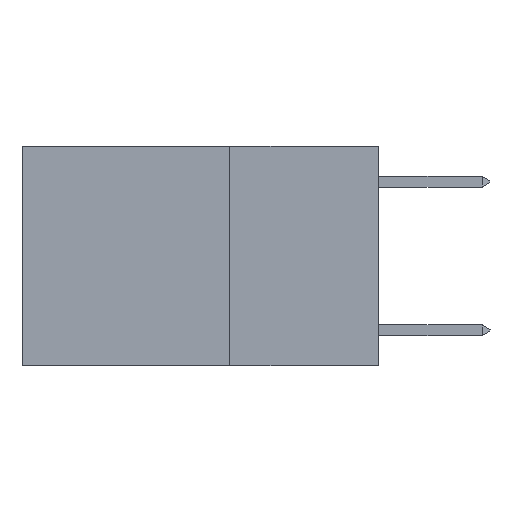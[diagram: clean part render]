
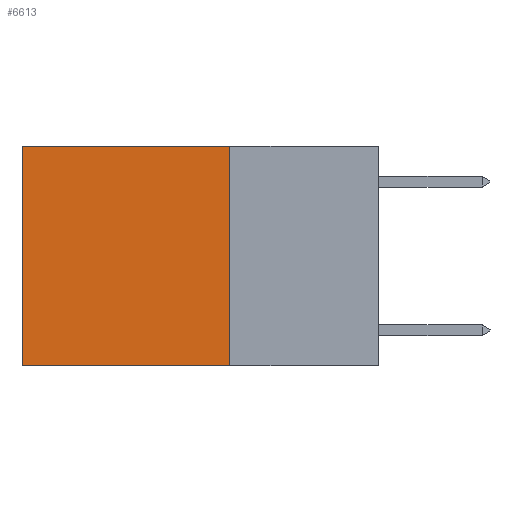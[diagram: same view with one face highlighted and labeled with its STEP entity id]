
A CAD part, left-side view. The second image highlights one B-rep face of the part: STEP entity #6613.
In plain terms, the highlighted planar face has unit normal (-1, 0, 0).
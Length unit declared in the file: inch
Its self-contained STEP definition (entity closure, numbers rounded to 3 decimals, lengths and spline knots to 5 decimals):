
#536 = EDGE_CURVE ( 'NONE', #12545, #14057, #3298, .T. ) ;
#821 = FACE_OUTER_BOUND ( 'NONE', #10818, .T. ) ;
#903 = EDGE_CURVE ( 'NONE', #1958, #10976, #19101, .T. ) ;
#1027 = EDGE_CURVE ( 'NONE', #12545, #1958, #18067, .T. ) ;
#1888 = ORIENTED_EDGE ( 'NONE', *, *, #536, .F. ) ;
#1958 = VERTEX_POINT ( 'NONE', #10747 ) ;
#2351 = ORIENTED_EDGE ( 'NONE', *, *, #14251, .F. ) ;
#2869 = VECTOR ( 'NONE', #5388, 39.37008 ) ;
#3298 = LINE ( 'NONE', #4580, #2869 ) ;
#4580 = CARTESIAN_POINT ( 'NONE',  ( 0.2625, 0.25, 0. ) ) ;
#5266 = CARTESIAN_POINT ( 'NONE',  ( 0.2625, 0.25, 0. ) ) ;
#5388 = DIRECTION ( 'NONE',  ( 0., 0., -1. ) ) ;
#6613 = ADVANCED_FACE ( 'NONE', ( #821 ), #17254, .F. ) ;
#7417 = CARTESIAN_POINT ( 'NONE',  ( 0.2625, 0.25, -0.37 ) ) ;
#7453 = ORIENTED_EDGE ( 'NONE', *, *, #1027, .T. ) ;
#10724 = AXIS2_PLACEMENT_3D ( 'NONE', #18256, #16936, #16872 ) ;
#10747 = CARTESIAN_POINT ( 'NONE',  ( 0.2625, 0.6, 0. ) ) ;
#10818 = EDGE_LOOP ( 'NONE', ( #18969, #2351, #1888, #7453 ) ) ;
#10976 = VERTEX_POINT ( 'NONE', #14517 ) ;
#11444 = CARTESIAN_POINT ( 'NONE',  ( 0.2625, 0.25, -0.37 ) ) ;
#11497 = DIRECTION ( 'NONE',  ( 0., 1., 0. ) ) ;
#11735 = CARTESIAN_POINT ( 'NONE',  ( 0.2625, 0.25, 0. ) ) ;
#11893 = DIRECTION ( 'NONE',  ( 0., 1., 0. ) ) ;
#12545 = VERTEX_POINT ( 'NONE', #5266 ) ;
#14057 = VERTEX_POINT ( 'NONE', #11444 ) ;
#14251 = EDGE_CURVE ( 'NONE', #14057, #10976, #17532, .T. ) ;
#14275 = CARTESIAN_POINT ( 'NONE',  ( 0.2625, 0.6, 0. ) ) ;
#14517 = CARTESIAN_POINT ( 'NONE',  ( 0.2625, 0.6, -0.37 ) ) ;
#14725 = DIRECTION ( 'NONE',  ( 0., 0., -1. ) ) ;
#16872 = DIRECTION ( 'NONE',  ( 0., 0., -1. ) ) ;
#16936 = DIRECTION ( 'NONE',  ( 1., 0., 0. ) ) ;
#17254 = PLANE ( 'NONE',  #10724 ) ;
#17473 = VECTOR ( 'NONE', #11893, 39.37008 ) ;
#17532 = LINE ( 'NONE', #7417, #17473 ) ;
#17961 = VECTOR ( 'NONE', #11497, 39.37008 ) ;
#18067 = LINE ( 'NONE', #11735, #17961 ) ;
#18256 = CARTESIAN_POINT ( 'NONE',  ( 0.2625, 0.25, 0. ) ) ;
#18484 = VECTOR ( 'NONE', #14725, 39.37008 ) ;
#18969 = ORIENTED_EDGE ( 'NONE', *, *, #903, .T. ) ;
#19101 = LINE ( 'NONE', #14275, #18484 ) ;
